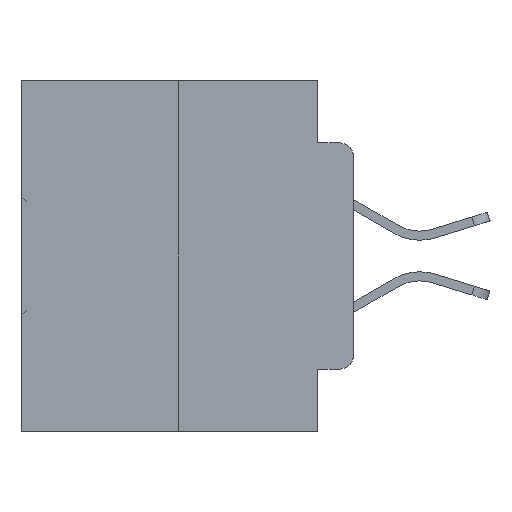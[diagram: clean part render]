
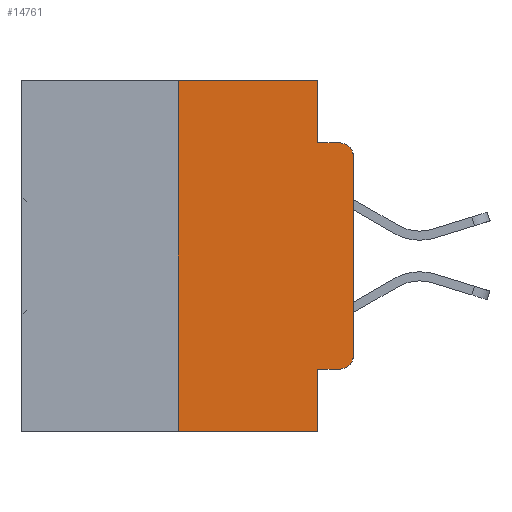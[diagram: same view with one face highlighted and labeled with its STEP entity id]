
A CAD part, left-side view. The second image highlights one B-rep face of the part: STEP entity #14761.
In plain terms, the highlighted planar face has unit normal (-1, 0, 0).
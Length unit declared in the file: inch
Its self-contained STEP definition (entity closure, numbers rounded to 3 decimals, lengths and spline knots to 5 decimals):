
#253 = ORIENTED_EDGE ( 'NONE', *, *, #19487, .T. ) ;
#596 = DIRECTION ( 'NONE',  ( -1., 0., 0. ) ) ;
#906 = ORIENTED_EDGE ( 'NONE', *, *, #6835, .T. ) ;
#1292 = CARTESIAN_POINT ( 'NONE',  ( 0., 0.051, -0.0885 ) ) ;
#1382 = ORIENTED_EDGE ( 'NONE', *, *, #12528, .T. ) ;
#1543 = ORIENTED_EDGE ( 'NONE', *, *, #20766, .F. ) ;
#2009 = VECTOR ( 'NONE', #29331, 39.37008 ) ;
#2271 = VECTOR ( 'NONE', #14306, 39.37008 ) ;
#2613 = ORIENTED_EDGE ( 'NONE', *, *, #14935, .F. ) ;
#2853 = LINE ( 'NONE', #11181, #9762 ) ;
#3112 = LINE ( 'NONE', #1292, #2271 ) ;
#3677 = ORIENTED_EDGE ( 'NONE', *, *, #22055, .F. ) ;
#3917 = FACE_OUTER_BOUND ( 'NONE', #12082, .T. ) ;
#4139 = VECTOR ( 'NONE', #14900, 39.37008 ) ;
#4505 = LINE ( 'NONE', #26729, #2009 ) ;
#5177 = VERTEX_POINT ( 'NONE', #17487 ) ;
#6247 = VERTEX_POINT ( 'NONE', #32379 ) ;
#6725 = CARTESIAN_POINT ( 'NONE',  ( 0., 0.473, 0. ) ) ;
#6835 = EDGE_CURVE ( 'NONE', #31077, #5177, #16324, .T. ) ;
#8466 = CARTESIAN_POINT ( 'NONE',  ( 0., 0.051, -0.4115 ) ) ;
#9195 = VERTEX_POINT ( 'NONE', #31476 ) ;
#9295 = DIRECTION ( 'NONE',  ( 0., 0., -1. ) ) ;
#9762 = VECTOR ( 'NONE', #31886, 39.37008 ) ;
#10165 = CARTESIAN_POINT ( 'NONE',  ( 0., 0.051, -0.5 ) ) ;
#11181 = CARTESIAN_POINT ( 'NONE',  ( 0., 0.473, -0.5 ) ) ;
#11211 = VECTOR ( 'NONE', #15121, 39.37008 ) ;
#11348 = CARTESIAN_POINT ( 'NONE',  ( 0., 0.02, -0.4115 ) ) ;
#11361 = VECTOR ( 'NONE', #32190, 39.37008 ) ;
#11904 = AXIS2_PLACEMENT_3D ( 'NONE', #13797, #31877, #16463 ) ;
#11958 = VERTEX_POINT ( 'NONE', #27427 ) ;
#12082 = EDGE_LOOP ( 'NONE', ( #906, #17114, #3677, #13809, #13237, #1543, #13331, #2613, #1382, #253 ) ) ;
#12273 = CARTESIAN_POINT ( 'NONE',  ( 0., 0.051, 0. ) ) ;
#12332 = EDGE_CURVE ( 'NONE', #11958, #33360, #2853, .T. ) ;
#12341 = EDGE_CURVE ( 'NONE', #6247, #9195, #4505, .T. ) ;
#12528 = EDGE_CURVE ( 'NONE', #17956, #21393, #23990, .T. ) ;
#13237 = ORIENTED_EDGE ( 'NONE', *, *, #12341, .F. ) ;
#13331 = ORIENTED_EDGE ( 'NONE', *, *, #12332, .T. ) ;
#13797 = CARTESIAN_POINT ( 'NONE',  ( 0., 0.02, -0.1085 ) ) ;
#13809 = ORIENTED_EDGE ( 'NONE', *, *, #19691, .F. ) ;
#14306 = DIRECTION ( 'NONE',  ( 0., -1., 0. ) ) ;
#14619 = VERTEX_POINT ( 'NONE', #24200 ) ;
#14761 = ADVANCED_FACE ( 'NONE', ( #3917 ), #22247, .F. ) ;
#14900 = DIRECTION ( 'NONE',  ( 0., 0., -1. ) ) ;
#14935 = EDGE_CURVE ( 'NONE', #17956, #33360, #18955, .T. ) ;
#15121 = DIRECTION ( 'NONE',  ( 0., 0., -1. ) ) ;
#15237 = CARTESIAN_POINT ( 'NONE',  ( 0., 0.051, 0. ) ) ;
#16295 = CARTESIAN_POINT ( 'NONE',  ( 0., 0.02, -0.3915 ) ) ;
#16324 = LINE ( 'NONE', #26971, #31632 ) ;
#16463 = DIRECTION ( 'NONE',  ( 0., 0., -1. ) ) ;
#16611 = DIRECTION ( 'NONE',  ( 0., 0., 1. ) ) ;
#17114 = ORIENTED_EDGE ( 'NONE', *, *, #29633, .T. ) ;
#17441 = AXIS2_PLACEMENT_3D ( 'NONE', #16295, #596, #18859 ) ;
#17487 = CARTESIAN_POINT ( 'NONE',  ( 0., 0., -0.1085 ) ) ;
#17956 = VERTEX_POINT ( 'NONE', #8466 ) ;
#17979 = LINE ( 'NONE', #12273, #4139 ) ;
#18859 = DIRECTION ( 'NONE',  ( 0., 0., -1. ) ) ;
#18955 = LINE ( 'NONE', #15237, #11211 ) ;
#19487 = EDGE_CURVE ( 'NONE', #21393, #31077, #31309, .T. ) ;
#19691 = EDGE_CURVE ( 'NONE', #9195, #14619, #17979, .T. ) ;
#20766 = EDGE_CURVE ( 'NONE', #11958, #6247, #25202, .T. ) ;
#21393 = VERTEX_POINT ( 'NONE', #11348 ) ;
#22055 = EDGE_CURVE ( 'NONE', #14619, #25622, #3112, .T. ) ;
#22089 = CARTESIAN_POINT ( 'NONE',  ( 0., 0., -0.3915 ) ) ;
#22247 = PLANE ( 'NONE',  #27736 ) ;
#22419 = CARTESIAN_POINT ( 'NONE',  ( 0., 0.051, -0.4115 ) ) ;
#23176 = VECTOR ( 'NONE', #25041, 39.37008 ) ;
#23781 = CIRCLE ( 'NONE', #11904, 0.02 ) ;
#23990 = LINE ( 'NONE', #22419, #23176 ) ;
#24200 = CARTESIAN_POINT ( 'NONE',  ( 0., 0.051, -0.0885 ) ) ;
#24874 = DIRECTION ( 'NONE',  ( 1., 0., 0. ) ) ;
#25041 = DIRECTION ( 'NONE',  ( 0., -1., 0. ) ) ;
#25202 = LINE ( 'NONE', #29634, #11361 ) ;
#25622 = VERTEX_POINT ( 'NONE', #31674 ) ;
#26729 = CARTESIAN_POINT ( 'NONE',  ( 0., 0.473, 0. ) ) ;
#26971 = CARTESIAN_POINT ( 'NONE',  ( 0., 0., 0. ) ) ;
#27427 = CARTESIAN_POINT ( 'NONE',  ( 0., 0.25, -0.5 ) ) ;
#27736 = AXIS2_PLACEMENT_3D ( 'NONE', #6725, #24874, #9295 ) ;
#29331 = DIRECTION ( 'NONE',  ( 0., -1., 0. ) ) ;
#29633 = EDGE_CURVE ( 'NONE', #5177, #25622, #23781, .T. ) ;
#29634 = CARTESIAN_POINT ( 'NONE',  ( 0., 0.25, 0. ) ) ;
#31077 = VERTEX_POINT ( 'NONE', #22089 ) ;
#31309 = CIRCLE ( 'NONE', #17441, 0.02 ) ;
#31476 = CARTESIAN_POINT ( 'NONE',  ( 0., 0.051, 0. ) ) ;
#31632 = VECTOR ( 'NONE', #16611, 39.37008 ) ;
#31674 = CARTESIAN_POINT ( 'NONE',  ( 0., 0.02, -0.0885 ) ) ;
#31877 = DIRECTION ( 'NONE',  ( -1., 0., 0. ) ) ;
#31886 = DIRECTION ( 'NONE',  ( 0., -1., 0. ) ) ;
#32190 = DIRECTION ( 'NONE',  ( 0., 0., 1. ) ) ;
#32379 = CARTESIAN_POINT ( 'NONE',  ( 0., 0.25, 0. ) ) ;
#33360 = VERTEX_POINT ( 'NONE', #10165 ) ;
